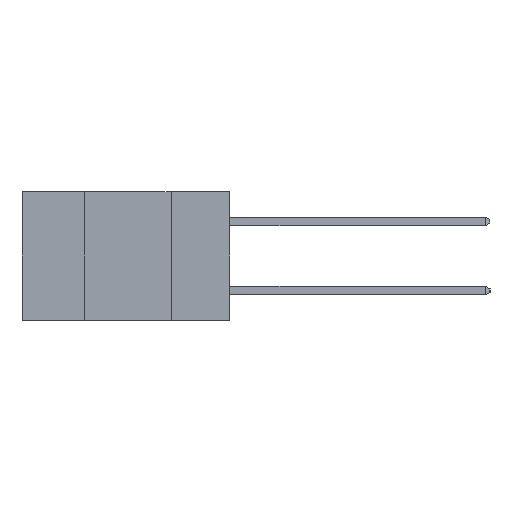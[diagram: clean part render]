
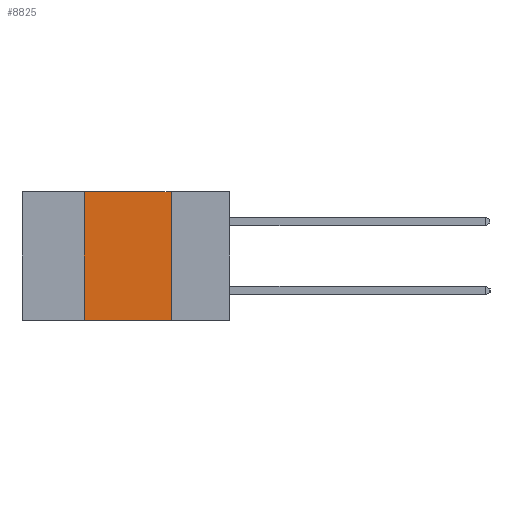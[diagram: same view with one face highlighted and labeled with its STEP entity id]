
A CAD part, left-side view. The second image highlights one B-rep face of the part: STEP entity #8825.
In plain terms, the highlighted planar face has unit normal (-1, 0, 0).
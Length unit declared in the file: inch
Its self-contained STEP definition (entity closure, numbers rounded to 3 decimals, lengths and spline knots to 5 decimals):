
#241 = EDGE_LOOP ( 'NONE', ( #646, #3801, #2817, #5768 ) ) ;
#449 = DIRECTION ( 'NONE',  ( 0., 0., -1. ) ) ;
#493 = LINE ( 'NONE', #7438, #9705 ) ;
#646 = ORIENTED_EDGE ( 'NONE', *, *, #7634, .F. ) ;
#1044 = EDGE_CURVE ( 'NONE', #5844, #7805, #493, .T. ) ;
#1507 = VECTOR ( 'NONE', #449, 39.37008 ) ;
#1517 = CARTESIAN_POINT ( 'NONE',  ( 0., 0.17, 0. ) ) ;
#1871 = VERTEX_POINT ( 'NONE', #5654 ) ;
#2544 = DIRECTION ( 'NONE',  ( 0., 0., 1. ) ) ;
#2636 = VERTEX_POINT ( 'NONE', #3136 ) ;
#2817 = ORIENTED_EDGE ( 'NONE', *, *, #10830, .F. ) ;
#3136 = CARTESIAN_POINT ( 'NONE',  ( 0., 0.42, -0.37 ) ) ;
#3564 = VECTOR ( 'NONE', #2544, 39.37008 ) ;
#3801 = ORIENTED_EDGE ( 'NONE', *, *, #1044, .F. ) ;
#3853 = VECTOR ( 'NONE', #7122, 39.37008 ) ;
#4333 = CARTESIAN_POINT ( 'NONE',  ( 0., 0.42, -0.37 ) ) ;
#4584 = CARTESIAN_POINT ( 'NONE',  ( 0., 0.6, 0. ) ) ;
#5307 = CARTESIAN_POINT ( 'NONE',  ( 0., 0.6, -0.37 ) ) ;
#5492 = DIRECTION ( 'NONE',  ( 0., 0., -1. ) ) ;
#5654 = CARTESIAN_POINT ( 'NONE',  ( 0., 0.17, -0.37 ) ) ;
#5768 = ORIENTED_EDGE ( 'NONE', *, *, #9713, .T. ) ;
#5844 = VERTEX_POINT ( 'NONE', #11423 ) ;
#5872 = DIRECTION ( 'NONE',  ( 0., -1., 0. ) ) ;
#6522 = AXIS2_PLACEMENT_3D ( 'NONE', #4584, #10862, #5492 ) ;
#7122 = DIRECTION ( 'NONE',  ( 0., -1., 0. ) ) ;
#7438 = CARTESIAN_POINT ( 'NONE',  ( 0., 0.6, 0. ) ) ;
#7634 = EDGE_CURVE ( 'NONE', #7805, #1871, #8637, .T. ) ;
#7805 = VERTEX_POINT ( 'NONE', #1517 ) ;
#8372 = LINE ( 'NONE', #4333, #3564 ) ;
#8637 = LINE ( 'NONE', #11134, #1507 ) ;
#8825 = ADVANCED_FACE ( 'NONE', ( #10193 ), #9084, .F. ) ;
#9084 = PLANE ( 'NONE',  #6522 ) ;
#9705 = VECTOR ( 'NONE', #5872, 39.37008 ) ;
#9713 = EDGE_CURVE ( 'NONE', #2636, #1871, #10435, .T. ) ;
#10193 = FACE_OUTER_BOUND ( 'NONE', #241, .T. ) ;
#10435 = LINE ( 'NONE', #5307, #3853 ) ;
#10830 = EDGE_CURVE ( 'NONE', #2636, #5844, #8372, .T. ) ;
#10862 = DIRECTION ( 'NONE',  ( 1., 0., 0. ) ) ;
#11134 = CARTESIAN_POINT ( 'NONE',  ( 0., 0.17, -0.37 ) ) ;
#11423 = CARTESIAN_POINT ( 'NONE',  ( 0., 0.42, 0. ) ) ;
